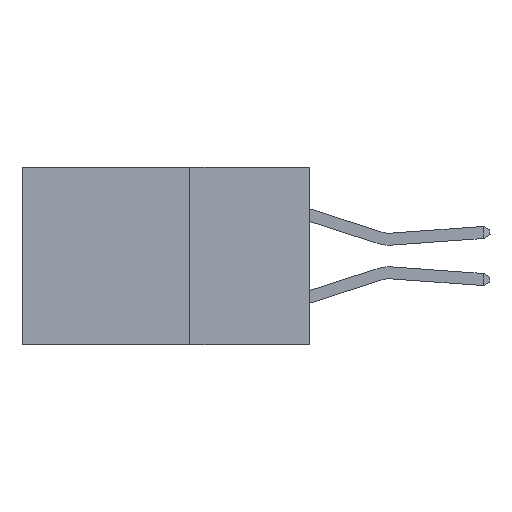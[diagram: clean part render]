
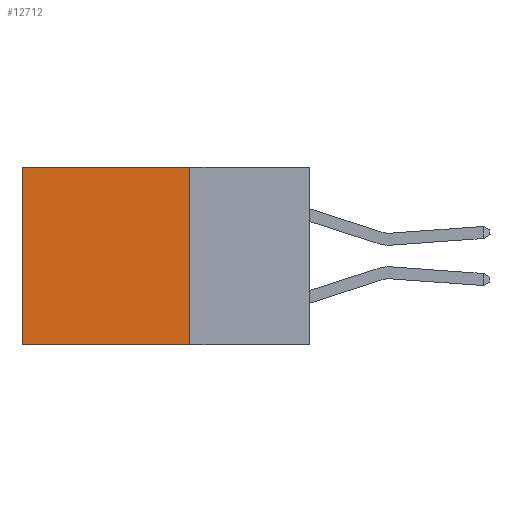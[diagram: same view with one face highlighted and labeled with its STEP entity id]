
A CAD part, left-side view. The second image highlights one B-rep face of the part: STEP entity #12712.
In plain terms, the highlighted planar face has unit normal (-1, 0, 0).
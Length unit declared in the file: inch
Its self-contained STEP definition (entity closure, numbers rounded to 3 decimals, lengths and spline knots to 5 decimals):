
#53 = VERTEX_POINT ( 'NONE', #6402 ) ;
#632 = VECTOR ( 'NONE', #4332, 39.37008 ) ;
#640 = CARTESIAN_POINT ( 'NONE',  ( 0.2615, 0.25, -0.37 ) ) ;
#736 = CARTESIAN_POINT ( 'NONE',  ( 0.2615, 0.25, -0.37 ) ) ;
#822 = CARTESIAN_POINT ( 'NONE',  ( 0.2615, 0.6, -0.37 ) ) ;
#847 = VECTOR ( 'NONE', #11979, 39.37008 ) ;
#1182 = LINE ( 'NONE', #640, #847 ) ;
#2068 = EDGE_LOOP ( 'NONE', ( #9394, #6765, #4357, #5118 ) ) ;
#2159 = VERTEX_POINT ( 'NONE', #10199 ) ;
#2723 = DIRECTION ( 'NONE',  ( 1., 0., 0. ) ) ;
#3286 = EDGE_CURVE ( 'NONE', #5881, #11540, #8939, .T. ) ;
#3872 = CARTESIAN_POINT ( 'NONE',  ( 0.2615, 0.25, 0. ) ) ;
#4284 = CARTESIAN_POINT ( 'NONE',  ( 0.2615, 0.6, 0. ) ) ;
#4332 = DIRECTION ( 'NONE',  ( 0., 0., -1. ) ) ;
#4357 = ORIENTED_EDGE ( 'NONE', *, *, #11487, .F. ) ;
#4423 = VECTOR ( 'NONE', #8110, 39.37008 ) ;
#4587 = CARTESIAN_POINT ( 'NONE',  ( 0.2615, 0.6, -0.37 ) ) ;
#5118 = ORIENTED_EDGE ( 'NONE', *, *, #8043, .T. ) ;
#5881 = VERTEX_POINT ( 'NONE', #4284 ) ;
#5988 = VECTOR ( 'NONE', #7009, 39.37008 ) ;
#6315 = LINE ( 'NONE', #3872, #5988 ) ;
#6402 = CARTESIAN_POINT ( 'NONE',  ( 0.2615, 0.25, -0.37 ) ) ;
#6765 = ORIENTED_EDGE ( 'NONE', *, *, #9134, .F. ) ;
#7009 = DIRECTION ( 'NONE',  ( 0., 1., 0. ) ) ;
#7200 = LINE ( 'NONE', #736, #4423 ) ;
#8043 = EDGE_CURVE ( 'NONE', #2159, #5881, #6315, .T. ) ;
#8110 = DIRECTION ( 'NONE',  ( 0., 0., -1. ) ) ;
#8126 = FACE_OUTER_BOUND ( 'NONE', #2068, .T. ) ;
#8321 = AXIS2_PLACEMENT_3D ( 'NONE', #8903, #2723, #9958 ) ;
#8903 = CARTESIAN_POINT ( 'NONE',  ( 0.2615, 0.25, -0.37 ) ) ;
#8939 = LINE ( 'NONE', #4587, #632 ) ;
#8948 = PLANE ( 'NONE',  #8321 ) ;
#9134 = EDGE_CURVE ( 'NONE', #53, #11540, #1182, .T. ) ;
#9394 = ORIENTED_EDGE ( 'NONE', *, *, #3286, .T. ) ;
#9958 = DIRECTION ( 'NONE',  ( 0., 0., -1. ) ) ;
#10199 = CARTESIAN_POINT ( 'NONE',  ( 0.2615, 0.25, 0. ) ) ;
#11487 = EDGE_CURVE ( 'NONE', #2159, #53, #7200, .T. ) ;
#11540 = VERTEX_POINT ( 'NONE', #822 ) ;
#11979 = DIRECTION ( 'NONE',  ( 0., 1., 0. ) ) ;
#12712 = ADVANCED_FACE ( 'NONE', ( #8126 ), #8948, .F. ) ;
